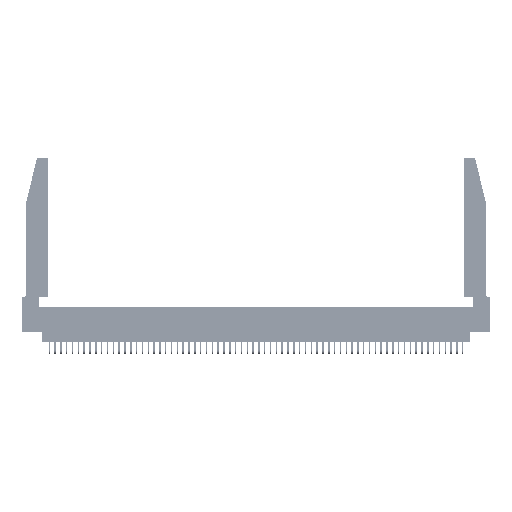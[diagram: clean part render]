
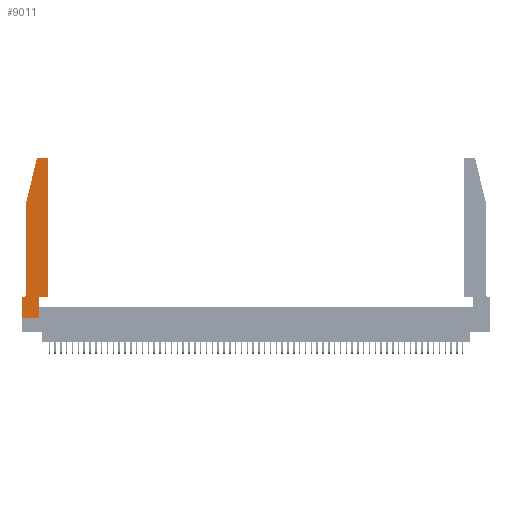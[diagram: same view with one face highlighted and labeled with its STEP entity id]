
A CAD part, top view. The second image highlights one B-rep face of the part: STEP entity #9011.
In plain terms, the highlighted planar face has unit normal (0, 0, 1).
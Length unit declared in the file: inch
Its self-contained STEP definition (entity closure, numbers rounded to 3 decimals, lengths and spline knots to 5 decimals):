
#707 = DIRECTION ( 'NONE',  ( 1., 0., 0. ) ) ;
#1676 = CARTESIAN_POINT ( 'NONE',  ( 0.0755, 2., 0.37 ) ) ;
#1677 = CIRCLE ( 'NONE', #16126, 0.07 ) ;
#1715 = CARTESIAN_POINT ( 'NONE',  ( 0.4505, 2.72, 0.37 ) ) ;
#2048 = EDGE_CURVE ( 'NONE', #15883, #30948, #54406, .T. ) ;
#2645 = VERTEX_POINT ( 'NONE', #54167 ) ;
#3628 = ORIENTED_EDGE ( 'NONE', *, *, #6851, .T. ) ;
#5711 = ORIENTED_EDGE ( 'NONE', *, *, #58713, .T. ) ;
#5963 = ORIENTED_EDGE ( 'NONE', *, *, #57583, .T. ) ;
#6851 = EDGE_CURVE ( 'NONE', #2645, #27464, #53561, .T. ) ;
#7003 = VECTOR ( 'NONE', #26733, 39.37008 ) ;
#7885 = VERTEX_POINT ( 'NONE', #55025 ) ;
#7955 = CIRCLE ( 'NONE', #22480, 0.03 ) ;
#9011 = ADVANCED_FACE ( 'NONE', ( #29216 ), #13906, .T. ) ;
#9498 = DIRECTION ( 'NONE',  ( 0., 0., 1. ) ) ;
#9644 = ORIENTED_EDGE ( 'NONE', *, *, #27805, .T. ) ;
#9902 = VERTEX_POINT ( 'NONE', #10412 ) ;
#10112 = VECTOR ( 'NONE', #45355, 39.37008 ) ;
#10412 = CARTESIAN_POINT ( 'NONE',  ( 0., 0., 0.37 ) ) ;
#11512 = ORIENTED_EDGE ( 'NONE', *, *, #15910, .T. ) ;
#11694 = DIRECTION ( 'NONE',  ( 0., -1., 0. ) ) ;
#13906 = PLANE ( 'NONE',  #39838 ) ;
#15571 = EDGE_CURVE ( 'NONE', #30644, #55583, #7955, .T. ) ;
#15883 = VERTEX_POINT ( 'NONE', #1715 ) ;
#15910 = EDGE_CURVE ( 'NONE', #53388, #20156, #43610, .T. ) ;
#16105 = CARTESIAN_POINT ( 'NONE',  ( 0.4505, 0.35, 0.37 ) ) ;
#16126 = AXIS2_PLACEMENT_3D ( 'NONE', #53660, #31394, #21833 ) ;
#17186 = CARTESIAN_POINT ( 'NONE',  ( 0.4505, 0.35, 0.37 ) ) ;
#17613 = DIRECTION ( 'NONE',  ( 0., 1., 0. ) ) ;
#18087 = CARTESIAN_POINT ( 'NONE',  ( 0.0755, 0.35, 0.37 ) ) ;
#18226 = CARTESIAN_POINT ( 'NONE',  ( 0.4505, 0.35, 0.37 ) ) ;
#18720 = CARTESIAN_POINT ( 'NONE',  ( 0., 0.35, 0.37 ) ) ;
#19347 = CARTESIAN_POINT ( 'NONE',  ( 0.284, 2.75, 0.37 ) ) ;
#20156 = VERTEX_POINT ( 'NONE', #57042 ) ;
#20833 = VECTOR ( 'NONE', #11694, 39.37008 ) ;
#21365 = DIRECTION ( 'NONE',  ( 0., 0., 1. ) ) ;
#21780 = EDGE_CURVE ( 'NONE', #30948, #30644, #27867, .T. ) ;
#21833 = DIRECTION ( 'NONE',  ( -1., 0., 0. ) ) ;
#22131 = ORIENTED_EDGE ( 'NONE', *, *, #21780, .T. ) ;
#22234 = ORIENTED_EDGE ( 'NONE', *, *, #26826, .T. ) ;
#22480 = AXIS2_PLACEMENT_3D ( 'NONE', #48799, #21365, #26129 ) ;
#22503 = ORIENTED_EDGE ( 'NONE', *, *, #35467, .T. ) ;
#23336 = EDGE_LOOP ( 'NONE', ( #22131, #46588, #5963, #11512, #26618, #3628, #9644, #22234, #52454, #22503, #5711, #42375 ) ) ;
#25111 = CARTESIAN_POINT ( 'NONE',  ( 0.0755, 2., 0.37 ) ) ;
#25238 = DIRECTION ( 'NONE',  ( -1., 0., 0. ) ) ;
#26129 = DIRECTION ( 'NONE',  ( 1., 0., 0. ) ) ;
#26618 = ORIENTED_EDGE ( 'NONE', *, *, #45220, .T. ) ;
#26733 = DIRECTION ( 'NONE',  ( 0., 1., 0. ) ) ;
#26826 = EDGE_CURVE ( 'NONE', #9902, #41161, #32628, .T. ) ;
#26965 = CARTESIAN_POINT ( 'NONE',  ( 0.2865, 0.35, 0.37 ) ) ;
#27279 = CARTESIAN_POINT ( 'NONE',  ( 0.0755, 2., 0.37 ) ) ;
#27464 = VERTEX_POINT ( 'NONE', #37769 ) ;
#27566 = DIRECTION ( 'NONE',  ( 1., 0., 0. ) ) ;
#27805 = EDGE_CURVE ( 'NONE', #27464, #9902, #31148, .T. ) ;
#27867 = LINE ( 'NONE', #37391, #54839 ) ;
#28184 = AXIS2_PLACEMENT_3D ( 'NONE', #31749, #36916, #27566 ) ;
#29216 = FACE_OUTER_BOUND ( 'NONE', #23336, .T. ) ;
#29766 = VECTOR ( 'NONE', #47142, 39.37008 ) ;
#30630 = LINE ( 'NONE', #17186, #7003 ) ;
#30644 = VERTEX_POINT ( 'NONE', #19347 ) ;
#30948 = VERTEX_POINT ( 'NONE', #39197 ) ;
#31148 = LINE ( 'NONE', #35128, #37551 ) ;
#31394 = DIRECTION ( 'NONE',  ( 0., 0., -1. ) ) ;
#31749 = CARTESIAN_POINT ( 'NONE',  ( 0.4205, 2.72, 0.37 ) ) ;
#32257 = DIRECTION ( 'NONE',  ( -0.239, -0.971, 0. ) ) ;
#32449 = CARTESIAN_POINT ( 'NONE',  ( 0., 0., 0.37 ) ) ;
#32628 = LINE ( 'NONE', #32449, #29766 ) ;
#33061 = CARTESIAN_POINT ( 'NONE',  ( 0.2865, 0., 0.37 ) ) ;
#34559 = VERTEX_POINT ( 'NONE', #16105 ) ;
#34777 = LINE ( 'NONE', #18226, #45476 ) ;
#35128 = CARTESIAN_POINT ( 'NONE',  ( 0., 0., 0.37 ) ) ;
#35467 = EDGE_CURVE ( 'NONE', #7885, #34559, #34777, .T. ) ;
#36916 = DIRECTION ( 'NONE',  ( 0., 0., 1. ) ) ;
#37391 = CARTESIAN_POINT ( 'NONE',  ( 0.2605, 2.75, 0.37 ) ) ;
#37551 = VECTOR ( 'NONE', #45076, 39.37008 ) ;
#37769 = CARTESIAN_POINT ( 'NONE',  ( 0., 0.35, 0.37 ) ) ;
#38565 = LINE ( 'NONE', #27279, #41450 ) ;
#39197 = CARTESIAN_POINT ( 'NONE',  ( 0.4205, 2.75, 0.37 ) ) ;
#39838 = AXIS2_PLACEMENT_3D ( 'NONE', #18720, #9498, #707 ) ;
#40312 = DIRECTION ( 'NONE',  ( 1., 0., 0. ) ) ;
#41161 = VERTEX_POINT ( 'NONE', #33061 ) ;
#41450 = VECTOR ( 'NONE', #32257, 39.37008 ) ;
#42304 = EDGE_CURVE ( 'NONE', #41161, #7885, #54093, .T. ) ;
#42375 = ORIENTED_EDGE ( 'NONE', *, *, #2048, .T. ) ;
#43610 = LINE ( 'NONE', #25111, #20833 ) ;
#45076 = DIRECTION ( 'NONE',  ( 0., -1., 0. ) ) ;
#45220 = EDGE_CURVE ( 'NONE', #20156, #2645, #1677, .T. ) ;
#45355 = DIRECTION ( 'NONE',  ( -1., 0., 0. ) ) ;
#45476 = VECTOR ( 'NONE', #40312, 39.37008 ) ;
#46588 = ORIENTED_EDGE ( 'NONE', *, *, #15571, .T. ) ;
#46730 = CARTESIAN_POINT ( 'NONE',  ( 0.25487, 2.72718, 0.37 ) ) ;
#47142 = DIRECTION ( 'NONE',  ( 1., 0., 0. ) ) ;
#48799 = CARTESIAN_POINT ( 'NONE',  ( 0.284, 2.72, 0.37 ) ) ;
#52454 = ORIENTED_EDGE ( 'NONE', *, *, #42304, .T. ) ;
#52661 = VECTOR ( 'NONE', #17613, 39.37008 ) ;
#53388 = VERTEX_POINT ( 'NONE', #1676 ) ;
#53561 = LINE ( 'NONE', #18087, #10112 ) ;
#53660 = CARTESIAN_POINT ( 'NONE',  ( 0.0055, 0.42, 0.37 ) ) ;
#54093 = LINE ( 'NONE', #26965, #52661 ) ;
#54167 = CARTESIAN_POINT ( 'NONE',  ( 0.0055, 0.35, 0.37 ) ) ;
#54406 = CIRCLE ( 'NONE', #28184, 0.03 ) ;
#54839 = VECTOR ( 'NONE', #25238, 39.37008 ) ;
#55025 = CARTESIAN_POINT ( 'NONE',  ( 0.2865, 0.35, 0.37 ) ) ;
#55583 = VERTEX_POINT ( 'NONE', #46730 ) ;
#57042 = CARTESIAN_POINT ( 'NONE',  ( 0.0755, 0.42, 0.37 ) ) ;
#57583 = EDGE_CURVE ( 'NONE', #55583, #53388, #38565, .T. ) ;
#58713 = EDGE_CURVE ( 'NONE', #34559, #15883, #30630, .T. ) ;
